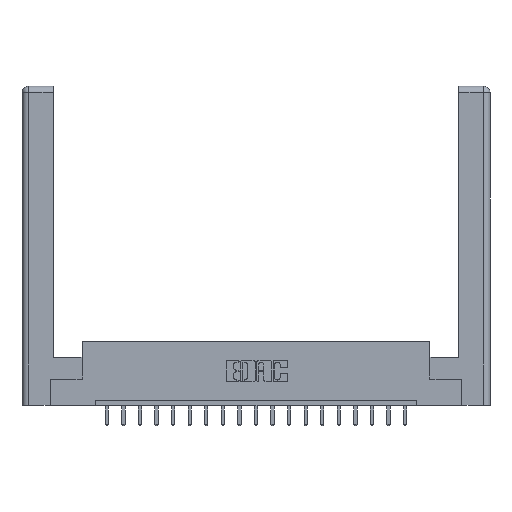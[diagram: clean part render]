
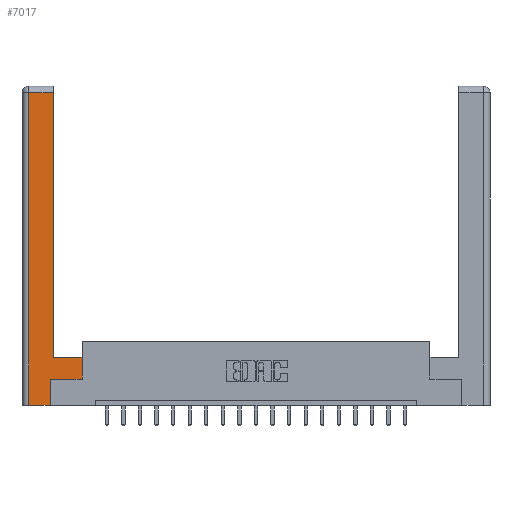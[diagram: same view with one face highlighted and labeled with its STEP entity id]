
A CAD part, top view. The second image highlights one B-rep face of the part: STEP entity #7017.
In plain terms, the highlighted planar face has unit normal (0, 0, 1).
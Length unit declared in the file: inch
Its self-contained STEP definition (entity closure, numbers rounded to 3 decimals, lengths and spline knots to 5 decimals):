
#90 = VECTOR ( 'NONE', #16086, 39.37008 ) ;
#319 = ORIENTED_EDGE ( 'NONE', *, *, #19403, .T. ) ;
#448 = VECTOR ( 'NONE', #17972, 39.37008 ) ;
#624 = CARTESIAN_POINT ( 'NONE',  ( 0.565, 0.245, 0. ) ) ;
#1157 = EDGE_LOOP ( 'NONE', ( #14519, #319, #6080, #9228, #6781, #5121, #19368, #6209 ) ) ;
#1238 = CARTESIAN_POINT ( 'NONE',  ( 0.0615, 2.94, 0. ) ) ;
#1520 = VERTEX_POINT ( 'NONE', #19250 ) ;
#2227 = PLANE ( 'NONE',  #16056 ) ;
#2387 = VERTEX_POINT ( 'NONE', #5661 ) ;
#2507 = CARTESIAN_POINT ( 'NONE',  ( 0.295, 2.94, 0. ) ) ;
#2898 = EDGE_CURVE ( 'NONE', #17268, #2387, #18142, .T. ) ;
#3679 = LINE ( 'NONE', #17932, #14754 ) ;
#3944 = CARTESIAN_POINT ( 'NONE',  ( 0.265, 0., 0. ) ) ;
#4902 = VECTOR ( 'NONE', #14169, 39.37008 ) ;
#5121 = ORIENTED_EDGE ( 'NONE', *, *, #18950, .T. ) ;
#5190 = CARTESIAN_POINT ( 'NONE',  ( 0.265, 0., 0. ) ) ;
#5285 = EDGE_CURVE ( 'NONE', #13871, #17268, #15000, .T. ) ;
#5307 = CARTESIAN_POINT ( 'NONE',  ( 0., 0., 0. ) ) ;
#5500 = DIRECTION ( 'NONE',  ( 1., 0., 0. ) ) ;
#5559 = EDGE_CURVE ( 'NONE', #1520, #19000, #3679, .T. ) ;
#5661 = CARTESIAN_POINT ( 'NONE',  ( 0.265, 0.245, 0. ) ) ;
#6080 = ORIENTED_EDGE ( 'NONE', *, *, #9008, .T. ) ;
#6209 = ORIENTED_EDGE ( 'NONE', *, *, #7309, .T. ) ;
#6582 = CARTESIAN_POINT ( 'NONE',  ( 0.265, 0.245, 0. ) ) ;
#6781 = ORIENTED_EDGE ( 'NONE', *, *, #2898, .T. ) ;
#6854 = LINE ( 'NONE', #18213, #16986 ) ;
#7017 = ADVANCED_FACE ( 'NONE', ( #7261 ), #2227, .F. ) ;
#7261 = FACE_OUTER_BOUND ( 'NONE', #1157, .T. ) ;
#7309 = EDGE_CURVE ( 'NONE', #11658, #1520, #14730, .T. ) ;
#7916 = VECTOR ( 'NONE', #12776, 39.37008 ) ;
#8397 = DIRECTION ( 'NONE',  ( -1., 0., 0. ) ) ;
#9008 = EDGE_CURVE ( 'NONE', #15352, #13871, #16597, .T. ) ;
#9016 = DIRECTION ( 'NONE',  ( 0., 1., 0. ) ) ;
#9228 = ORIENTED_EDGE ( 'NONE', *, *, #5285, .T. ) ;
#10434 = VERTEX_POINT ( 'NONE', #11106 ) ;
#10628 = EDGE_CURVE ( 'NONE', #10434, #11658, #6854, .T. ) ;
#10903 = VECTOR ( 'NONE', #5500, 39.37008 ) ;
#11106 = CARTESIAN_POINT ( 'NONE',  ( 0.565, 0.245, 0. ) ) ;
#11562 = DIRECTION ( 'NONE',  ( 0., 1., 0. ) ) ;
#11658 = VERTEX_POINT ( 'NONE', #13038 ) ;
#12066 = CARTESIAN_POINT ( 'NONE',  ( 0.0615, 0., 0. ) ) ;
#12776 = DIRECTION ( 'NONE',  ( -1., 0., 0. ) ) ;
#13038 = CARTESIAN_POINT ( 'NONE',  ( 0.565, 0.45, 0. ) ) ;
#13350 = CARTESIAN_POINT ( 'NONE',  ( 0.0615, 0., 0. ) ) ;
#13871 = VERTEX_POINT ( 'NONE', #12066 ) ;
#14169 = DIRECTION ( 'NONE',  ( 0., 1., 0. ) ) ;
#14519 = ORIENTED_EDGE ( 'NONE', *, *, #5559, .T. ) ;
#14730 = LINE ( 'NONE', #16626, #15667 ) ;
#14754 = VECTOR ( 'NONE', #11562, 39.37008 ) ;
#15000 = LINE ( 'NONE', #3944, #10903 ) ;
#15352 = VERTEX_POINT ( 'NONE', #1238 ) ;
#15667 = VECTOR ( 'NONE', #18270, 39.37008 ) ;
#15924 = CARTESIAN_POINT ( 'NONE',  ( 0.0615, 2.94, 0. ) ) ;
#16056 = AXIS2_PLACEMENT_3D ( 'NONE', #5307, #17608, #8397 ) ;
#16086 = DIRECTION ( 'NONE',  ( 1., 0., 0. ) ) ;
#16597 = LINE ( 'NONE', #13350, #448 ) ;
#16626 = CARTESIAN_POINT ( 'NONE',  ( 0.295, 0.45, 0. ) ) ;
#16986 = VECTOR ( 'NONE', #9016, 39.37008 ) ;
#17268 = VERTEX_POINT ( 'NONE', #5190 ) ;
#17311 = LINE ( 'NONE', #15924, #7916 ) ;
#17608 = DIRECTION ( 'NONE',  ( 0., 0., -1. ) ) ;
#17932 = CARTESIAN_POINT ( 'NONE',  ( 0.295, 3., 0. ) ) ;
#17972 = DIRECTION ( 'NONE',  ( 0., -1., 0. ) ) ;
#18142 = LINE ( 'NONE', #6582, #4902 ) ;
#18213 = CARTESIAN_POINT ( 'NONE',  ( 0.565, 0.45, 0. ) ) ;
#18270 = DIRECTION ( 'NONE',  ( -1., 0., 0. ) ) ;
#18805 = LINE ( 'NONE', #624, #90 ) ;
#18950 = EDGE_CURVE ( 'NONE', #2387, #10434, #18805, .T. ) ;
#19000 = VERTEX_POINT ( 'NONE', #2507 ) ;
#19250 = CARTESIAN_POINT ( 'NONE',  ( 0.295, 0.45, 0. ) ) ;
#19368 = ORIENTED_EDGE ( 'NONE', *, *, #10628, .T. ) ;
#19403 = EDGE_CURVE ( 'NONE', #19000, #15352, #17311, .T. ) ;
